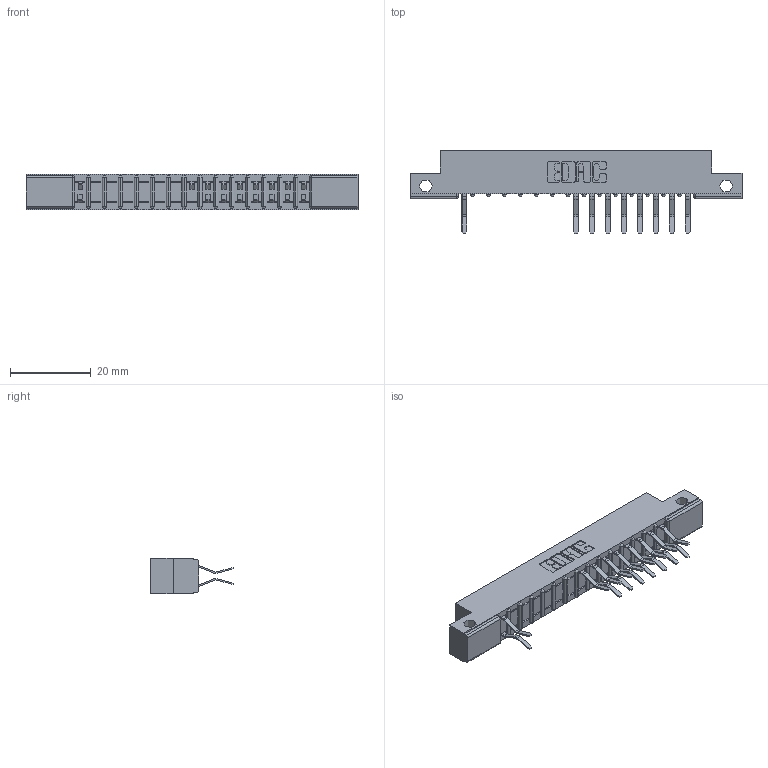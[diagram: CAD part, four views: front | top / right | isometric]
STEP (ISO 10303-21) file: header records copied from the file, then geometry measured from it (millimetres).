
FILE_DESCRIPTION (( 'STEP AP203' ), '1' );
FILE_NAME ('307-030-560-212.STEP', '2018-08-04T20:01:38', ( '' ), ( '' ), 'SwSTEP 2.0', 'SolidWorks 2016', '' );
FILE_SCHEMA (( 'CONFIG_CONTROL_DESIGN' ));
Length unit declared in the file: inch
Products named in the file (3): 307 Part_.128 Dia Side Mounting Holes; 307-290-001_560; 307-030-560-212
Assembly tree (18 placements, depth 2):
  307-030-560-212
    307 Part_.128 Dia Side Mounting Holes
    307-290-001_560  x17
Bounding box: 82.45 x 20.65 x 8.71 mm (x, y, z)
Volume: 241.3 mm3
Topology: 17 solids, 21 shells, 1114 faces, 3150 edges, 2031 vertices
Faces by surface type: plane 709, cylinder 373, sphere 32
Full cylindrical faces by diameter (mm): 1.016 x1
Entity records: 16352 total; most frequent: CARTESIAN_POINT 2738, ORIENTED_EDGE 2722, DIRECTION 2681, EDGE_CURVE 1358, LINE 1031, VECTOR 1031, VERTEX_POINT 882, AXIS2_PLACEMENT_3D 825
